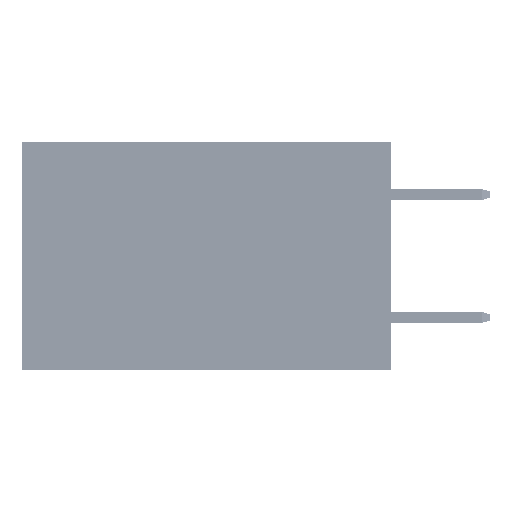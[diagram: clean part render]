
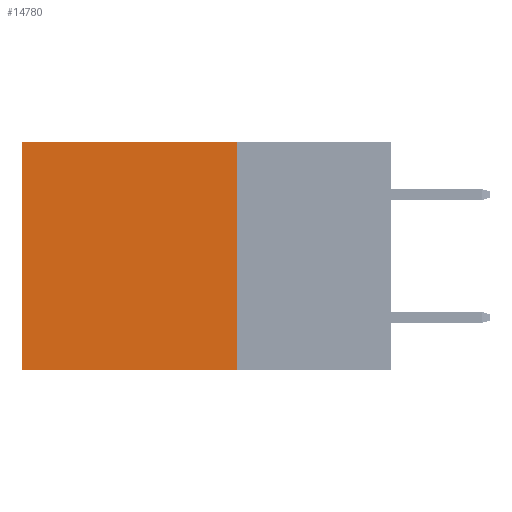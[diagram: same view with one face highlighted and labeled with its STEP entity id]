
A CAD part, left-side view. The second image highlights one B-rep face of the part: STEP entity #14780.
In plain terms, the highlighted planar face has unit normal (-1, 0, 0).
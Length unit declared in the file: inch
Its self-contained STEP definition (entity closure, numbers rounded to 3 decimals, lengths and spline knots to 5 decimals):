
#3171 = VECTOR ( 'NONE', #50362, 39.37008 ) ;
#4035 = CARTESIAN_POINT ( 'NONE',  ( 0.2875, 0.6, 0. ) ) ;
#7454 = CARTESIAN_POINT ( 'NONE',  ( 0.2875, 0.25, 0. ) ) ;
#7518 = LINE ( 'NONE', #31015, #41037 ) ;
#8737 = LINE ( 'NONE', #41131, #23590 ) ;
#8859 = ORIENTED_EDGE ( 'NONE', *, *, #18428, .T. ) ;
#10606 = VERTEX_POINT ( 'NONE', #45995 ) ;
#12526 = ORIENTED_EDGE ( 'NONE', *, *, #21871, .F. ) ;
#12784 = ORIENTED_EDGE ( 'NONE', *, *, #16171, .T. ) ;
#13886 = LINE ( 'NONE', #32953, #41809 ) ;
#13984 = CARTESIAN_POINT ( 'NONE',  ( 0.2875, 0.25, 0. ) ) ;
#14780 = ADVANCED_FACE ( 'NONE', ( #37740 ), #17642, .F. ) ;
#16171 = EDGE_CURVE ( 'NONE', #43264, #21758, #34871, .T. ) ;
#17642 = PLANE ( 'NONE',  #38189 ) ;
#18428 = EDGE_CURVE ( 'NONE', #21758, #20108, #7518, .T. ) ;
#20108 = VERTEX_POINT ( 'NONE', #46695 ) ;
#21758 = VERTEX_POINT ( 'NONE', #4035 ) ;
#21871 = EDGE_CURVE ( 'NONE', #10606, #20108, #8737, .T. ) ;
#23590 = VECTOR ( 'NONE', #24142, 39.37008 ) ;
#23689 = DIRECTION ( 'NONE',  ( 0., 0., -1. ) ) ;
#24142 = DIRECTION ( 'NONE',  ( 0., 1., 0. ) ) ;
#25107 = DIRECTION ( 'NONE',  ( 0., 0., -1. ) ) ;
#29396 = DIRECTION ( 'NONE',  ( 0., 0., -1. ) ) ;
#29901 = DIRECTION ( 'NONE',  ( 1., 0., 0. ) ) ;
#31015 = CARTESIAN_POINT ( 'NONE',  ( 0.2875, 0.6, 0. ) ) ;
#32637 = EDGE_LOOP ( 'NONE', ( #8859, #12526, #48505, #12784 ) ) ;
#32953 = CARTESIAN_POINT ( 'NONE',  ( 0.2875, 0.25, 0. ) ) ;
#33284 = EDGE_CURVE ( 'NONE', #43264, #10606, #13886, .T. ) ;
#34871 = LINE ( 'NONE', #7454, #3171 ) ;
#37411 = CARTESIAN_POINT ( 'NONE',  ( 0.2875, 0.25, 0. ) ) ;
#37740 = FACE_OUTER_BOUND ( 'NONE', #32637, .T. ) ;
#38189 = AXIS2_PLACEMENT_3D ( 'NONE', #13984, #29901, #29396 ) ;
#41037 = VECTOR ( 'NONE', #23689, 39.37008 ) ;
#41131 = CARTESIAN_POINT ( 'NONE',  ( 0.2875, 0.25, -0.37 ) ) ;
#41809 = VECTOR ( 'NONE', #25107, 39.37008 ) ;
#43264 = VERTEX_POINT ( 'NONE', #37411 ) ;
#45995 = CARTESIAN_POINT ( 'NONE',  ( 0.2875, 0.25, -0.37 ) ) ;
#46695 = CARTESIAN_POINT ( 'NONE',  ( 0.2875, 0.6, -0.37 ) ) ;
#48505 = ORIENTED_EDGE ( 'NONE', *, *, #33284, .F. ) ;
#50362 = DIRECTION ( 'NONE',  ( 0., 1., 0. ) ) ;
